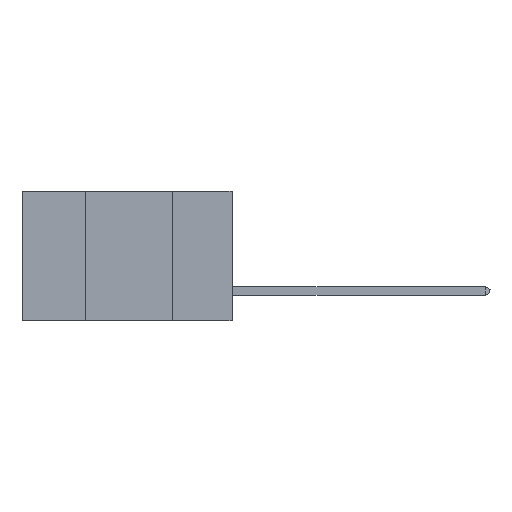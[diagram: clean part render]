
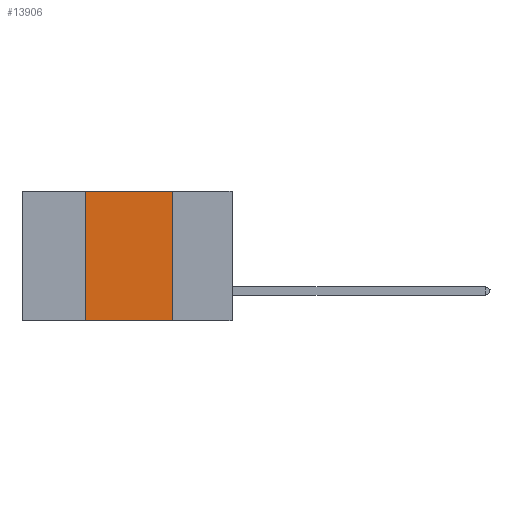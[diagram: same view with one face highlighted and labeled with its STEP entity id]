
A CAD part, left-side view. The second image highlights one B-rep face of the part: STEP entity #13906.
In plain terms, the highlighted planar face has unit normal (-1, 0, 0).
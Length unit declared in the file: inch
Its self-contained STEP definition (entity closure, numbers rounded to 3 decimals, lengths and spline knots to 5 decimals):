
#58 = ORIENTED_EDGE ( 'NONE', *, *, #2904, .T. ) ;
#328 = DIRECTION ( 'NONE',  ( 0., -1., 0. ) ) ;
#1046 = LINE ( 'NONE', #8845, #16467 ) ;
#1771 = DIRECTION ( 'NONE',  ( 0., 0., -1. ) ) ;
#1834 = PLANE ( 'NONE',  #16420 ) ;
#2904 = EDGE_CURVE ( 'NONE', #13774, #11355, #1046, .T. ) ;
#3007 = LINE ( 'NONE', #19217, #11854 ) ;
#3135 = EDGE_LOOP ( 'NONE', ( #17634, #8435, #14645, #58 ) ) ;
#3347 = CARTESIAN_POINT ( 'NONE',  ( 0., 0.6, 0. ) ) ;
#4682 = DIRECTION ( 'NONE',  ( 1., 0., 0. ) ) ;
#4757 = VECTOR ( 'NONE', #328, 39.37008 ) ;
#5242 = EDGE_CURVE ( 'NONE', #13774, #16659, #3007, .T. ) ;
#5790 = CARTESIAN_POINT ( 'NONE',  ( 0., 0.17, 0. ) ) ;
#6148 = CARTESIAN_POINT ( 'NONE',  ( 0., 0.42, 0. ) ) ;
#6707 = LINE ( 'NONE', #5790, #10476 ) ;
#8435 = ORIENTED_EDGE ( 'NONE', *, *, #19098, .F. ) ;
#8845 = CARTESIAN_POINT ( 'NONE',  ( 0., 0.6, -0.37 ) ) ;
#9409 = LINE ( 'NONE', #3347, #4757 ) ;
#10039 = CARTESIAN_POINT ( 'NONE',  ( 0., 0.17, 0. ) ) ;
#10476 = VECTOR ( 'NONE', #17865, 39.37008 ) ;
#10747 = CARTESIAN_POINT ( 'NONE',  ( 0., 0.6, 0. ) ) ;
#11355 = VERTEX_POINT ( 'NONE', #11908 ) ;
#11854 = VECTOR ( 'NONE', #13201, 39.37008 ) ;
#11907 = DIRECTION ( 'NONE',  ( 0., -1., 0. ) ) ;
#11908 = CARTESIAN_POINT ( 'NONE',  ( 0., 0.17, -0.37 ) ) ;
#13201 = DIRECTION ( 'NONE',  ( 0., 0., 1. ) ) ;
#13774 = VERTEX_POINT ( 'NONE', #14171 ) ;
#13906 = ADVANCED_FACE ( 'NONE', ( #18462 ), #1834, .F. ) ;
#14171 = CARTESIAN_POINT ( 'NONE',  ( 0., 0.42, -0.37 ) ) ;
#14645 = ORIENTED_EDGE ( 'NONE', *, *, #5242, .F. ) ;
#15348 = EDGE_CURVE ( 'NONE', #17082, #11355, #6707, .T. ) ;
#16420 = AXIS2_PLACEMENT_3D ( 'NONE', #10747, #4682, #1771 ) ;
#16467 = VECTOR ( 'NONE', #11907, 39.37008 ) ;
#16659 = VERTEX_POINT ( 'NONE', #6148 ) ;
#17082 = VERTEX_POINT ( 'NONE', #10039 ) ;
#17634 = ORIENTED_EDGE ( 'NONE', *, *, #15348, .F. ) ;
#17865 = DIRECTION ( 'NONE',  ( 0., 0., -1. ) ) ;
#18462 = FACE_OUTER_BOUND ( 'NONE', #3135, .T. ) ;
#19098 = EDGE_CURVE ( 'NONE', #16659, #17082, #9409, .T. ) ;
#19217 = CARTESIAN_POINT ( 'NONE',  ( 0., 0.42, 0. ) ) ;
